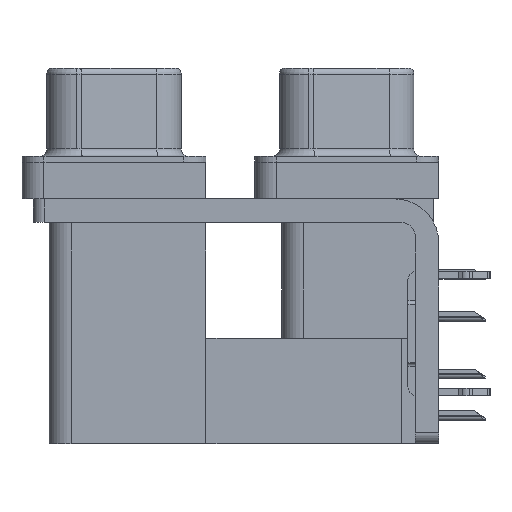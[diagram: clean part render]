
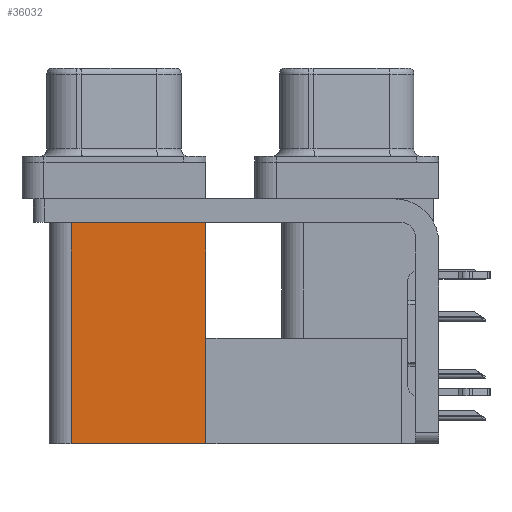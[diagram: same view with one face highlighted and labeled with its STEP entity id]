
A CAD part, left-side view. The second image highlights one B-rep face of the part: STEP entity #36032.
In plain terms, the highlighted planar face has unit normal (-1, 0, 0).
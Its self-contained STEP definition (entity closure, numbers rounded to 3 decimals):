
#377 = CARTESIAN_POINT ( 'NONE',  ( 3.7, 9.6, -2.5 ) ) ;
#390 = CARTESIAN_POINT ( 'NONE',  ( 3.7, 9.6, -2.5 ) ) ;
#610 = DIRECTION ( 'NONE',  ( 0., 1., 0. ) ) ;
#2226 = DIRECTION ( 'NONE',  ( 1., 0., 0. ) ) ;
#3503 = EDGE_LOOP ( 'NONE', ( #4153, #10938, #38441, #27716 ) ) ;
#4153 = ORIENTED_EDGE ( 'NONE', *, *, #32373, .T. ) ;
#5731 = CARTESIAN_POINT ( 'NONE',  ( 3.7, 9.6, -19.2 ) ) ;
#6708 = VERTEX_POINT ( 'NONE', #377 ) ;
#7437 = LINE ( 'NONE', #19871, #24912 ) ;
#10107 = CARTESIAN_POINT ( 'NONE',  ( 3.7, 18.8, -19.2 ) ) ;
#10938 = ORIENTED_EDGE ( 'NONE', *, *, #42115, .F. ) ;
#10995 = VECTOR ( 'NONE', #25320, 1000. ) ;
#11003 = VERTEX_POINT ( 'NONE', #10107 ) ;
#15248 = CARTESIAN_POINT ( 'NONE',  ( 3.7, 18.8, -2.5 ) ) ;
#15755 = LINE ( 'NONE', #25536, #40178 ) ;
#15913 = VECTOR ( 'NONE', #610, 1000. ) ;
#18759 = PLANE ( 'NONE',  #22970 ) ;
#19024 = LINE ( 'NONE', #5731, #10995 ) ;
#19673 = DIRECTION ( 'NONE',  ( 0., 1., 0. ) ) ;
#19871 = CARTESIAN_POINT ( 'NONE',  ( 3.7, 18.8, -19.2 ) ) ;
#20408 = LINE ( 'NONE', #390, #15913 ) ;
#20617 = VERTEX_POINT ( 'NONE', #15248 ) ;
#22224 = DIRECTION ( 'NONE',  ( 0., 0., -1. ) ) ;
#22970 = AXIS2_PLACEMENT_3D ( 'NONE', #32017, #2226, #22224 ) ;
#24912 = VECTOR ( 'NONE', #36800, 1000. ) ;
#25320 = DIRECTION ( 'NONE',  ( 0., 0., 1. ) ) ;
#25536 = CARTESIAN_POINT ( 'NONE',  ( 3.7, 9.6, -19.2 ) ) ;
#27716 = ORIENTED_EDGE ( 'NONE', *, *, #41768, .T. ) ;
#32017 = CARTESIAN_POINT ( 'NONE',  ( 3.7, 9.6, -19.2 ) ) ;
#32373 = EDGE_CURVE ( 'NONE', #6708, #20617, #20408, .T. ) ;
#34030 = CARTESIAN_POINT ( 'NONE',  ( 3.7, 9.6, -19.2 ) ) ;
#35257 = FACE_OUTER_BOUND ( 'NONE', #3503, .T. ) ;
#36032 = ADVANCED_FACE ( 'NONE', ( #35257 ), #18759, .F. ) ;
#36724 = VERTEX_POINT ( 'NONE', #34030 ) ;
#36800 = DIRECTION ( 'NONE',  ( 0., 0., 1. ) ) ;
#38441 = ORIENTED_EDGE ( 'NONE', *, *, #41959, .F. ) ;
#40178 = VECTOR ( 'NONE', #19673, 1000. ) ;
#41768 = EDGE_CURVE ( 'NONE', #36724, #6708, #19024, .T. ) ;
#41959 = EDGE_CURVE ( 'NONE', #36724, #11003, #15755, .T. ) ;
#42115 = EDGE_CURVE ( 'NONE', #11003, #20617, #7437, .T. ) ;
